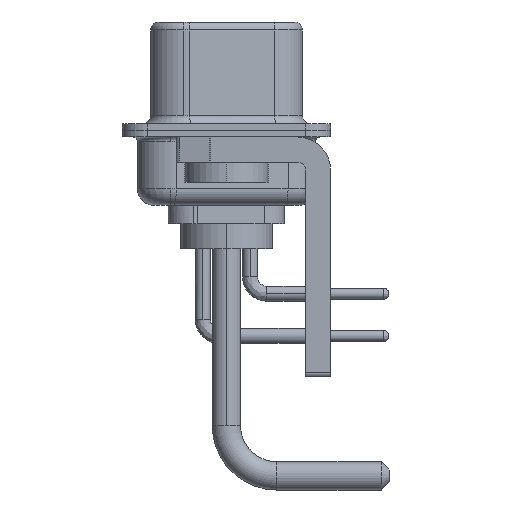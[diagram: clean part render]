
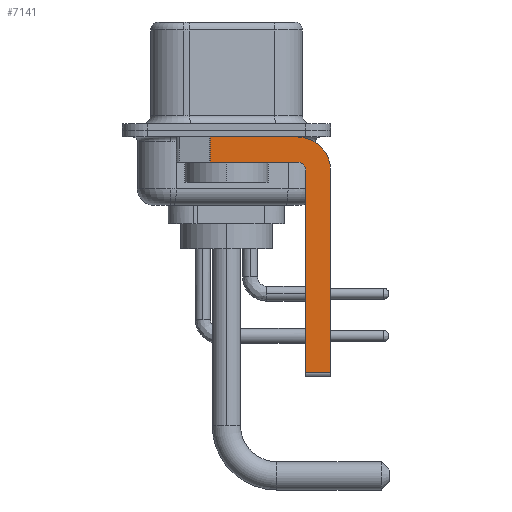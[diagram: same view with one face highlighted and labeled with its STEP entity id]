
A CAD part, left-side view. The second image highlights one B-rep face of the part: STEP entity #7141.
In plain terms, the highlighted planar face has unit normal (-1, 0, 0).
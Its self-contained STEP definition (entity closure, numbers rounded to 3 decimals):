
#181 = ORIENTED_EDGE ( 'NONE', *, *, #16657, .T. ) ;
#243 = EDGE_LOOP ( 'NONE', ( #22472, #926, #1622, #10359, #15955, #181, #12765, #12273 ) ) ;
#465 = LINE ( 'NONE', #6079, #3319 ) ;
#591 = DIRECTION ( 'NONE',  ( 1., 0., 0. ) ) ;
#916 = CARTESIAN_POINT ( 'NONE',  ( -2.9, -4.75, -2.4 ) ) ;
#926 = ORIENTED_EDGE ( 'NONE', *, *, #22742, .T. ) ;
#1250 = DIRECTION ( 'NONE',  ( 0., -1., 0. ) ) ;
#1622 = ORIENTED_EDGE ( 'NONE', *, *, #3348, .F. ) ;
#2417 = VERTEX_POINT ( 'NONE', #24296 ) ;
#3319 = VECTOR ( 'NONE', #12577, 1000. ) ;
#3348 = EDGE_CURVE ( 'NONE', #12408, #14071, #6547, .T. ) ;
#3367 = DIRECTION ( 'NONE',  ( -1., 0., 0. ) ) ;
#5091 = DIRECTION ( 'NONE',  ( 1., 0., 0. ) ) ;
#6079 = CARTESIAN_POINT ( 'NONE',  ( -2.9, 0.978, -1.9 ) ) ;
#6547 = LINE ( 'NONE', #24071, #25476 ) ;
#7014 = LINE ( 'NONE', #13129, #22786 ) ;
#7141 = ADVANCED_FACE ( 'NONE', ( #22867 ), #8715, .F. ) ;
#7205 = VERTEX_POINT ( 'NONE', #916 ) ;
#7598 = CARTESIAN_POINT ( 'NONE',  ( -2.9, -6.25, -2.4 ) ) ;
#7733 = EDGE_CURVE ( 'NONE', #21960, #14874, #7983, .T. ) ;
#7983 = LINE ( 'NONE', #7598, #25400 ) ;
#8530 = DIRECTION ( 'NONE',  ( 0., 0., -1. ) ) ;
#8592 = CARTESIAN_POINT ( 'NONE',  ( -2.9, -4.75, -14.55 ) ) ;
#8715 = PLANE ( 'NONE',  #17788 ) ;
#9621 = VERTEX_POINT ( 'NONE', #8592 ) ;
#9955 = CIRCLE ( 'NONE', #11618, 2. ) ;
#10321 = EDGE_CURVE ( 'NONE', #7205, #12408, #14743, .T. ) ;
#10359 = ORIENTED_EDGE ( 'NONE', *, *, #10321, .F. ) ;
#10580 = AXIS2_PLACEMENT_3D ( 'NONE', #13257, #3367, #11308 ) ;
#10632 = VERTEX_POINT ( 'NONE', #15049 ) ;
#10940 = CARTESIAN_POINT ( 'NONE',  ( -2.9, -4.25, -2.4 ) ) ;
#11308 = DIRECTION ( 'NONE',  ( 0., 0., 1. ) ) ;
#11419 = CARTESIAN_POINT ( 'NONE',  ( -2.9, -4.25, -1.9 ) ) ;
#11618 = AXIS2_PLACEMENT_3D ( 'NONE', #12439, #591, #8530 ) ;
#12046 = CARTESIAN_POINT ( 'NONE',  ( -2.9, 0.978, -1.9 ) ) ;
#12273 = ORIENTED_EDGE ( 'NONE', *, *, #22837, .F. ) ;
#12370 = CARTESIAN_POINT ( 'NONE',  ( -2.9, -6.25, -2.4 ) ) ;
#12408 = VERTEX_POINT ( 'NONE', #11419 ) ;
#12439 = CARTESIAN_POINT ( 'NONE',  ( -2.9, -4.25, -2.4 ) ) ;
#12577 = DIRECTION ( 'NONE',  ( 0., 0., -1. ) ) ;
#12765 = ORIENTED_EDGE ( 'NONE', *, *, #7733, .F. ) ;
#13129 = CARTESIAN_POINT ( 'NONE',  ( -2.9, -4.75, -14.8 ) ) ;
#13257 = CARTESIAN_POINT ( 'NONE',  ( -2.9, -4.25, -2.4 ) ) ;
#13835 = DIRECTION ( 'NONE',  ( 0., -1., 0. ) ) ;
#14071 = VERTEX_POINT ( 'NONE', #12046 ) ;
#14743 = CIRCLE ( 'NONE', #10580, 0.5 ) ;
#14746 = DIRECTION ( 'NONE',  ( 0., 1., 0. ) ) ;
#14874 = VERTEX_POINT ( 'NONE', #20328 ) ;
#15049 = CARTESIAN_POINT ( 'NONE',  ( -2.9, 0.978, -0.4 ) ) ;
#15174 = CARTESIAN_POINT ( 'NONE',  ( -2.9, 3., -0.4 ) ) ;
#15705 = VECTOR ( 'NONE', #13835, 1000. ) ;
#15955 = ORIENTED_EDGE ( 'NONE', *, *, #22459, .F. ) ;
#16033 = CARTESIAN_POINT ( 'NONE',  ( -2.9, -4.25, -14.55 ) ) ;
#16657 = EDGE_CURVE ( 'NONE', #9621, #14874, #23544, .T. ) ;
#17788 = AXIS2_PLACEMENT_3D ( 'NONE', #10940, #5091, #22997 ) ;
#20328 = CARTESIAN_POINT ( 'NONE',  ( -2.9, -6.25, -14.55 ) ) ;
#20619 = LINE ( 'NONE', #15174, #24943 ) ;
#21032 = DIRECTION ( 'NONE',  ( 0., 0., 1. ) ) ;
#21960 = VERTEX_POINT ( 'NONE', #12370 ) ;
#22459 = EDGE_CURVE ( 'NONE', #9621, #7205, #7014, .T. ) ;
#22472 = ORIENTED_EDGE ( 'NONE', *, *, #24060, .F. ) ;
#22742 = EDGE_CURVE ( 'NONE', #10632, #14071, #465, .T. ) ;
#22786 = VECTOR ( 'NONE', #21032, 1000. ) ;
#22837 = EDGE_CURVE ( 'NONE', #2417, #21960, #9955, .T. ) ;
#22867 = FACE_OUTER_BOUND ( 'NONE', #243, .T. ) ;
#22997 = DIRECTION ( 'NONE',  ( 0., 0., -1. ) ) ;
#23544 = LINE ( 'NONE', #16033, #15705 ) ;
#24060 = EDGE_CURVE ( 'NONE', #10632, #2417, #20619, .T. ) ;
#24071 = CARTESIAN_POINT ( 'NONE',  ( -2.9, -4.25, -1.9 ) ) ;
#24296 = CARTESIAN_POINT ( 'NONE',  ( -2.9, -4.25, -0.4 ) ) ;
#24943 = VECTOR ( 'NONE', #1250, 1000. ) ;
#25400 = VECTOR ( 'NONE', #25507, 1000. ) ;
#25476 = VECTOR ( 'NONE', #14746, 1000. ) ;
#25507 = DIRECTION ( 'NONE',  ( 0., 0., -1. ) ) ;
